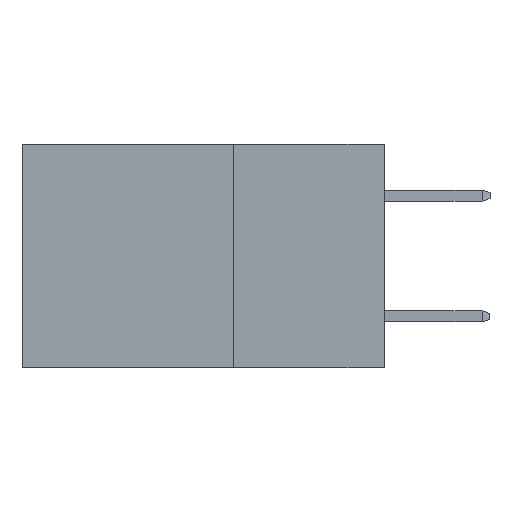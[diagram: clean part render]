
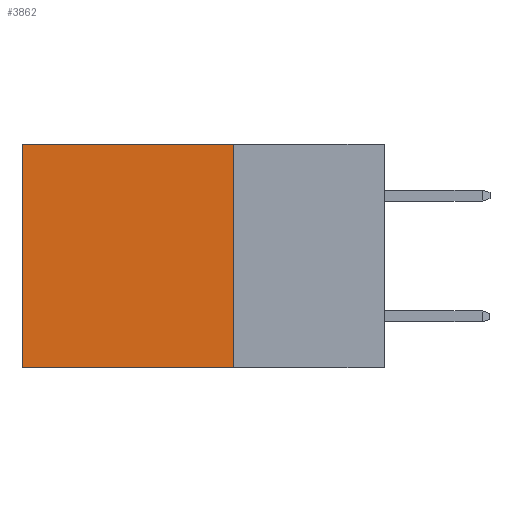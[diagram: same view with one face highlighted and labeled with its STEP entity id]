
A CAD part, left-side view. The second image highlights one B-rep face of the part: STEP entity #3862.
In plain terms, the highlighted planar face has unit normal (-1, 0, 0).
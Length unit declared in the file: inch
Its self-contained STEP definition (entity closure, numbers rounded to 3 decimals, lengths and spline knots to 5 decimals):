
#385 = EDGE_CURVE ( 'NONE', #7889, #787, #9387, .T. ) ;
#543 = ORIENTED_EDGE ( 'NONE', *, *, #2327, .T. ) ;
#787 = VERTEX_POINT ( 'NONE', #4595 ) ;
#854 = CARTESIAN_POINT ( 'NONE',  ( 0.298, 0.6, 0. ) ) ;
#2024 = FACE_OUTER_BOUND ( 'NONE', #2536, .T. ) ;
#2061 = CARTESIAN_POINT ( 'NONE',  ( 0.298, 0.25, -0.37 ) ) ;
#2327 = EDGE_CURVE ( 'NONE', #787, #2801, #2944, .T. ) ;
#2525 = DIRECTION ( 'NONE',  ( 0., 0., -1. ) ) ;
#2536 = EDGE_LOOP ( 'NONE', ( #543, #5429, #11413, #11283 ) ) ;
#2801 = VERTEX_POINT ( 'NONE', #7658 ) ;
#2944 = LINE ( 'NONE', #854, #7469 ) ;
#3274 = DIRECTION ( 'NONE',  ( 0., 1., 0. ) ) ;
#3636 = LINE ( 'NONE', #9778, #10591 ) ;
#3862 = ADVANCED_FACE ( 'NONE', ( #2024 ), #10612, .F. ) ;
#4069 = DIRECTION ( 'NONE',  ( 0., 0., -1. ) ) ;
#4097 = CARTESIAN_POINT ( 'NONE',  ( 0.298, 0.25, 0. ) ) ;
#4332 = DIRECTION ( 'NONE',  ( 0., 0., -1. ) ) ;
#4546 = VECTOR ( 'NONE', #3274, 39.37008 ) ;
#4595 = CARTESIAN_POINT ( 'NONE',  ( 0.298, 0.6, 0. ) ) ;
#5272 = VERTEX_POINT ( 'NONE', #7770 ) ;
#5429 = ORIENTED_EDGE ( 'NONE', *, *, #6229, .F. ) ;
#6229 = EDGE_CURVE ( 'NONE', #5272, #2801, #9709, .T. ) ;
#7469 = VECTOR ( 'NONE', #2525, 39.37008 ) ;
#7635 = CARTESIAN_POINT ( 'NONE',  ( 0.298, 0.25, 0. ) ) ;
#7658 = CARTESIAN_POINT ( 'NONE',  ( 0.298, 0.6, -0.37 ) ) ;
#7770 = CARTESIAN_POINT ( 'NONE',  ( 0.298, 0.25, -0.37 ) ) ;
#7889 = VERTEX_POINT ( 'NONE', #7635 ) ;
#8485 = DIRECTION ( 'NONE',  ( 0., 1., 0. ) ) ;
#8852 = AXIS2_PLACEMENT_3D ( 'NONE', #4097, #10369, #4069 ) ;
#9387 = LINE ( 'NONE', #10890, #4546 ) ;
#9709 = LINE ( 'NONE', #2061, #11754 ) ;
#9778 = CARTESIAN_POINT ( 'NONE',  ( 0.298, 0.25, 0. ) ) ;
#10369 = DIRECTION ( 'NONE',  ( 1., 0., 0. ) ) ;
#10541 = EDGE_CURVE ( 'NONE', #7889, #5272, #3636, .T. ) ;
#10591 = VECTOR ( 'NONE', #4332, 39.37008 ) ;
#10612 = PLANE ( 'NONE',  #8852 ) ;
#10890 = CARTESIAN_POINT ( 'NONE',  ( 0.298, 0.25, 0. ) ) ;
#11283 = ORIENTED_EDGE ( 'NONE', *, *, #385, .T. ) ;
#11413 = ORIENTED_EDGE ( 'NONE', *, *, #10541, .F. ) ;
#11754 = VECTOR ( 'NONE', #8485, 39.37008 ) ;
